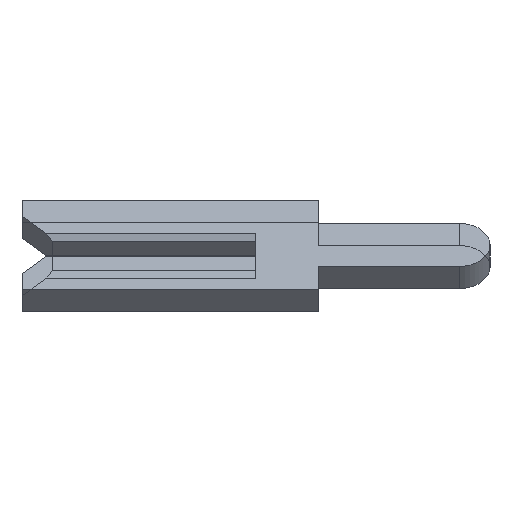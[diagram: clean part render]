
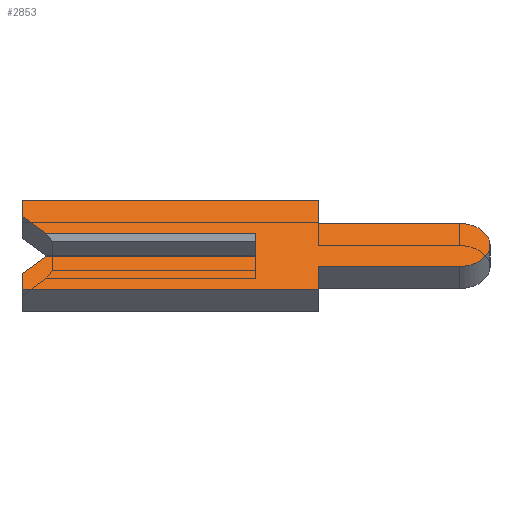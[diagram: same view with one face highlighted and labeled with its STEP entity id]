
A CAD part, left-side view. The second image highlights one B-rep face of the part: STEP entity #2853.
In plain terms, the highlighted face is planar.
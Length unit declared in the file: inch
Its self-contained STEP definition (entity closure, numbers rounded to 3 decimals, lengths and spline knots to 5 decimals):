
#9 = CARTESIAN_POINT ( 'NONE',  ( -0.01, 0.15, 0.026 ) ) ;
#16 = CARTESIAN_POINT ( 'NONE',  ( -0.01, -0.1305, 0. ) ) ;
#35 = VERTEX_POINT ( 'NONE', #2155 ) ;
#50 = EDGE_CURVE ( 'NONE', #521, #3142, #1017, .T. ) ;
#61 = CARTESIAN_POINT ( 'NONE',  ( -0.01, -0.04, 0.0195 ) ) ;
#82 = CARTESIAN_POINT ( 'NONE',  ( -0.01, 0.15, 0.026 ) ) ;
#141 = EDGE_CURVE ( 'NONE', #706, #3236, #293, .T. ) ;
#167 = EDGE_CURVE ( 'NONE', #35, #3384, #1911, .T. ) ;
#273 = DIRECTION ( 'NONE',  ( 1., 0., 0. ) ) ;
#293 = LINE ( 'NONE', #2701, #3396 ) ;
#343 = VERTEX_POINT ( 'NONE', #1105 ) ;
#354 = EDGE_CURVE ( 'NONE', #3384, #521, #1794, .T. ) ;
#369 = VECTOR ( 'NONE', #609, 39.37008 ) ;
#372 = EDGE_CURVE ( 'NONE', #1819, #2804, #1532, .T. ) ;
#521 = VERTEX_POINT ( 'NONE', #61 ) ;
#524 = EDGE_CURVE ( 'NONE', #1130, #2021, #2079, .T. ) ;
#576 = FACE_OUTER_BOUND ( 'NONE', #1314, .T. ) ;
#609 = DIRECTION ( 'NONE',  ( 0., 0., 1. ) ) ;
#633 = CARTESIAN_POINT ( 'NONE',  ( -0.01, -0.1305, 0.0195 ) ) ;
#706 = VERTEX_POINT ( 'NONE', #2458 ) ;
#724 = LINE ( 'NONE', #1983, #2702 ) ;
#744 = EDGE_CURVE ( 'NONE', #2846, #3158, #724, .T. ) ;
#781 = DIRECTION ( 'NONE',  ( 0., -1., 0. ) ) ;
#879 = DIRECTION ( 'NONE',  ( 0., 0., -1. ) ) ;
#892 = VECTOR ( 'NONE', #1358, 39.37008 ) ;
#908 = DIRECTION ( 'NONE',  ( 0., -1., 0. ) ) ;
#1017 = LINE ( 'NONE', #1346, #1565 ) ;
#1033 = VECTOR ( 'NONE', #2696, 39.37008 ) ;
#1039 = CARTESIAN_POINT ( 'NONE',  ( -0.01, 0.134, 0.01 ) ) ;
#1094 = LINE ( 'NONE', #1451, #369 ) ;
#1098 = DIRECTION ( 'NONE',  ( 0., 0., -1. ) ) ;
#1105 = CARTESIAN_POINT ( 'NONE',  ( -0.01, 0.134, -0.01 ) ) ;
#1130 = VERTEX_POINT ( 'NONE', #1722 ) ;
#1138 = VECTOR ( 'NONE', #2525, 39.37008 ) ;
#1216 = LINE ( 'NONE', #1671, #1033 ) ;
#1265 = ORIENTED_EDGE ( 'NONE', *, *, #3043, .F. ) ;
#1314 = EDGE_LOOP ( 'NONE', ( #1344, #3111, #2477, #2107, #3255, #2742, #1265, #1388, #1434, #2659, #3060, #2029, #2658, #2186 ) ) ;
#1344 = ORIENTED_EDGE ( 'NONE', *, *, #3459, .T. ) ;
#1346 = CARTESIAN_POINT ( 'NONE',  ( -0.01, -0.04, 0.0195 ) ) ;
#1358 = DIRECTION ( 'NONE',  ( 0., -1., 0. ) ) ;
#1367 = VECTOR ( 'NONE', #2770, 39.37008 ) ;
#1388 = ORIENTED_EDGE ( 'NONE', *, *, #141, .F. ) ;
#1407 = AXIS2_PLACEMENT_3D ( 'NONE', #1627, #273, #1098 ) ;
#1409 = CARTESIAN_POINT ( 'NONE',  ( -0.01, 0.1305, 0.0065 ) ) ;
#1417 = CARTESIAN_POINT ( 'NONE',  ( -0.01, -0.1305, -0.01 ) ) ;
#1430 = CARTESIAN_POINT ( 'NONE',  ( -0.01, -0.04, -0.04 ) ) ;
#1434 = ORIENTED_EDGE ( 'NONE', *, *, #2234, .F. ) ;
#1451 = CARTESIAN_POINT ( 'NONE',  ( -0.01, 0.15, -0.026 ) ) ;
#1532 = LINE ( 'NONE', #1409, #1827 ) ;
#1565 = VECTOR ( 'NONE', #781, 39.37008 ) ;
#1627 = CARTESIAN_POINT ( 'NONE',  ( -0.01, -0.1305, 0. ) ) ;
#1671 = CARTESIAN_POINT ( 'NONE',  ( -0.01, 0.1305, -0.0065 ) ) ;
#1722 = CARTESIAN_POINT ( 'NONE',  ( -0.01, -0.04, -0.04 ) ) ;
#1732 = VECTOR ( 'NONE', #908, 39.37008 ) ;
#1780 = VERTEX_POINT ( 'NONE', #2389 ) ;
#1794 = LINE ( 'NONE', #2226, #3022 ) ;
#1814 = LINE ( 'NONE', #1430, #2800 ) ;
#1819 = VERTEX_POINT ( 'NONE', #1039 ) ;
#1827 = VECTOR ( 'NONE', #2511, 39.37008 ) ;
#1875 = CARTESIAN_POINT ( 'NONE',  ( -0.01, 0.15, 0.04 ) ) ;
#1911 = LINE ( 'NONE', #1875, #892 ) ;
#1927 = CIRCLE ( 'NONE', #1407, 0.0195 ) ;
#1929 = DIRECTION ( 'NONE',  ( 1., 0., 0. ) ) ;
#1983 = CARTESIAN_POINT ( 'NONE',  ( -0.01, 0., 0.0065 ) ) ;
#2021 = VERTEX_POINT ( 'NONE', #3214 ) ;
#2029 = ORIENTED_EDGE ( 'NONE', *, *, #167, .F. ) ;
#2079 = LINE ( 'NONE', #2216, #1367 ) ;
#2107 = ORIENTED_EDGE ( 'NONE', *, *, #2427, .F. ) ;
#2155 = CARTESIAN_POINT ( 'NONE',  ( -0.01, 0.15, 0.04 ) ) ;
#2186 = ORIENTED_EDGE ( 'NONE', *, *, #372, .F. ) ;
#2216 = CARTESIAN_POINT ( 'NONE',  ( -0.01, 0.15, -0.04 ) ) ;
#2221 = CARTESIAN_POINT ( 'NONE',  ( -0.01, 0.15, 0.01 ) ) ;
#2226 = CARTESIAN_POINT ( 'NONE',  ( -0.01, -0.04, 0.04 ) ) ;
#2234 = EDGE_CURVE ( 'NONE', #3142, #706, #1927, .T. ) ;
#2389 = CARTESIAN_POINT ( 'NONE',  ( -0.01, 0.15, -0.026 ) ) ;
#2427 = EDGE_CURVE ( 'NONE', #1780, #343, #1216, .T. ) ;
#2458 = CARTESIAN_POINT ( 'NONE',  ( -0.01, -0.1305, -0.0195 ) ) ;
#2466 = DIRECTION ( 'NONE',  ( 0., 0., -1. ) ) ;
#2476 = CARTESIAN_POINT ( 'NONE',  ( -0.01, -0.04, -0.0195 ) ) ;
#2477 = ORIENTED_EDGE ( 'NONE', *, *, #3266, .F. ) ;
#2511 = DIRECTION ( 'NONE',  ( 0., 0.707, 0.707 ) ) ;
#2525 = DIRECTION ( 'NONE',  ( 0., 0., 1. ) ) ;
#2530 = AXIS2_PLACEMENT_3D ( 'NONE', #16, #1929, #2466 ) ;
#2576 = LINE ( 'NONE', #82, #1138 ) ;
#2658 = ORIENTED_EDGE ( 'NONE', *, *, #3439, .F. ) ;
#2659 = ORIENTED_EDGE ( 'NONE', *, *, #50, .F. ) ;
#2696 = DIRECTION ( 'NONE',  ( 0., -0.707, 0.707 ) ) ;
#2701 = CARTESIAN_POINT ( 'NONE',  ( -0.01, -0.04, -0.0195 ) ) ;
#2702 = VECTOR ( 'NONE', #2836, 39.37008 ) ;
#2703 = VECTOR ( 'NONE', #3350, 39.37008 ) ;
#2742 = ORIENTED_EDGE ( 'NONE', *, *, #524, .F. ) ;
#2770 = DIRECTION ( 'NONE',  ( 0., 1., 0. ) ) ;
#2779 = CARTESIAN_POINT ( 'NONE',  ( -0.01, -0.04, 0.04 ) ) ;
#2800 = VECTOR ( 'NONE', #2805, 39.37008 ) ;
#2804 = VERTEX_POINT ( 'NONE', #9 ) ;
#2805 = DIRECTION ( 'NONE',  ( 0., 0., -1. ) ) ;
#2836 = DIRECTION ( 'NONE',  ( 0., 0., 1. ) ) ;
#2846 = VERTEX_POINT ( 'NONE', #3314 ) ;
#2853 = ADVANCED_FACE ( 'NONE', ( #576 ), #3015, .F. ) ;
#2985 = DIRECTION ( 'NONE',  ( 0., 1., 0. ) ) ;
#3015 = PLANE ( 'NONE',  #2530 ) ;
#3022 = VECTOR ( 'NONE', #879, 39.37008 ) ;
#3043 = EDGE_CURVE ( 'NONE', #3236, #1130, #1814, .T. ) ;
#3060 = ORIENTED_EDGE ( 'NONE', *, *, #354, .F. ) ;
#3067 = EDGE_CURVE ( 'NONE', #2021, #1780, #1094, .T. ) ;
#3086 = CARTESIAN_POINT ( 'NONE',  ( -0.01, 0., 0.01 ) ) ;
#3111 = ORIENTED_EDGE ( 'NONE', *, *, #744, .F. ) ;
#3142 = VERTEX_POINT ( 'NONE', #633 ) ;
#3158 = VERTEX_POINT ( 'NONE', #3086 ) ;
#3214 = CARTESIAN_POINT ( 'NONE',  ( -0.01, 0.15, -0.04 ) ) ;
#3236 = VERTEX_POINT ( 'NONE', #2476 ) ;
#3255 = ORIENTED_EDGE ( 'NONE', *, *, #3067, .F. ) ;
#3266 = EDGE_CURVE ( 'NONE', #343, #2846, #3466, .T. ) ;
#3282 = LINE ( 'NONE', #2221, #2703 ) ;
#3314 = CARTESIAN_POINT ( 'NONE',  ( -0.01, 0., -0.01 ) ) ;
#3350 = DIRECTION ( 'NONE',  ( 0., -1., 0. ) ) ;
#3384 = VERTEX_POINT ( 'NONE', #2779 ) ;
#3396 = VECTOR ( 'NONE', #2985, 39.37008 ) ;
#3439 = EDGE_CURVE ( 'NONE', #2804, #35, #2576, .T. ) ;
#3459 = EDGE_CURVE ( 'NONE', #1819, #3158, #3282, .T. ) ;
#3466 = LINE ( 'NONE', #1417, #1732 ) ;
